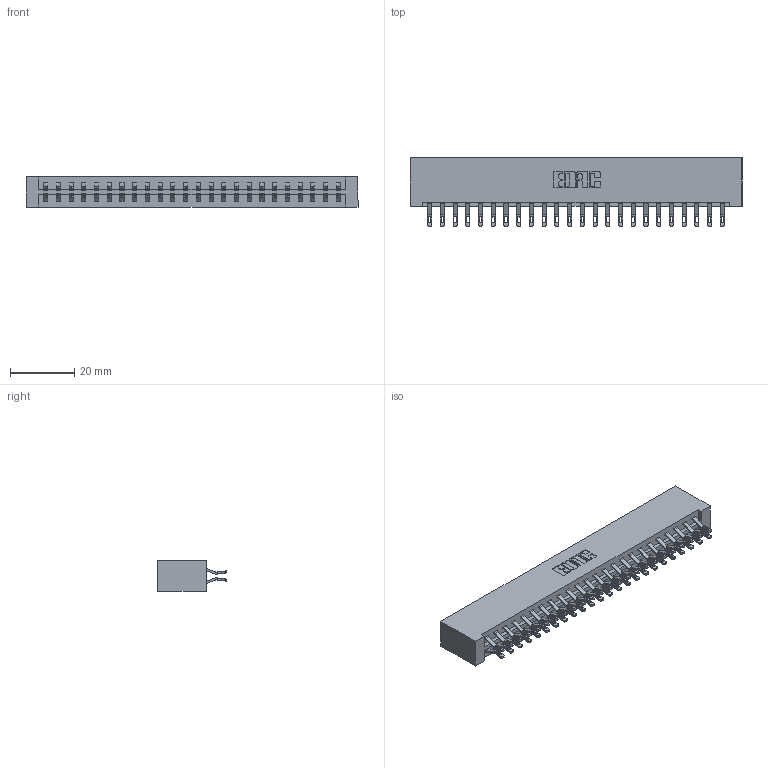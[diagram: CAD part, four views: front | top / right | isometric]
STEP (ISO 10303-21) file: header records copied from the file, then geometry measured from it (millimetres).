
FILE_DESCRIPTION (( 'STEP AP203' ), '1' );
FILE_NAME ('833-048-555-201.STEP', '2020-06-04T16:18:18', ( '' ), ( '' ), 'SwSTEP 2.0', 'SolidWorks 2020', '' );
FILE_SCHEMA (( 'CONFIG_CONTROL_DESIGN' ));
Length unit declared in the file: inch
Products named in the file (3): 833-048-555-201; 833 Part_Lugless; 345-292-001_555 Tail
Assembly tree (49 placements, depth 2):
  833-048-555-201
    833 Part_Lugless
    345-292-001_555 Tail  x48
Bounding box: 103.35 x 21.47 x 9.4 mm (x, y, z)
Volume: 11154.8 mm3; surface area: 13539.4 mm2
Topology: 49 solids, 49 shells, 2890 faces, 9071 edges, 6046 vertices
Faces by surface type: plane 1698, cylinder 1192
Entity records: 17817 total; most frequent: CARTESIAN_POINT 3008, ORIENTED_EDGE 2914, DIRECTION 2565, EDGE_CURVE 1457, VECTOR 1317, LINE 1317, VERTEX_POINT 970, AXIS2_PLACEMENT_3D 624
